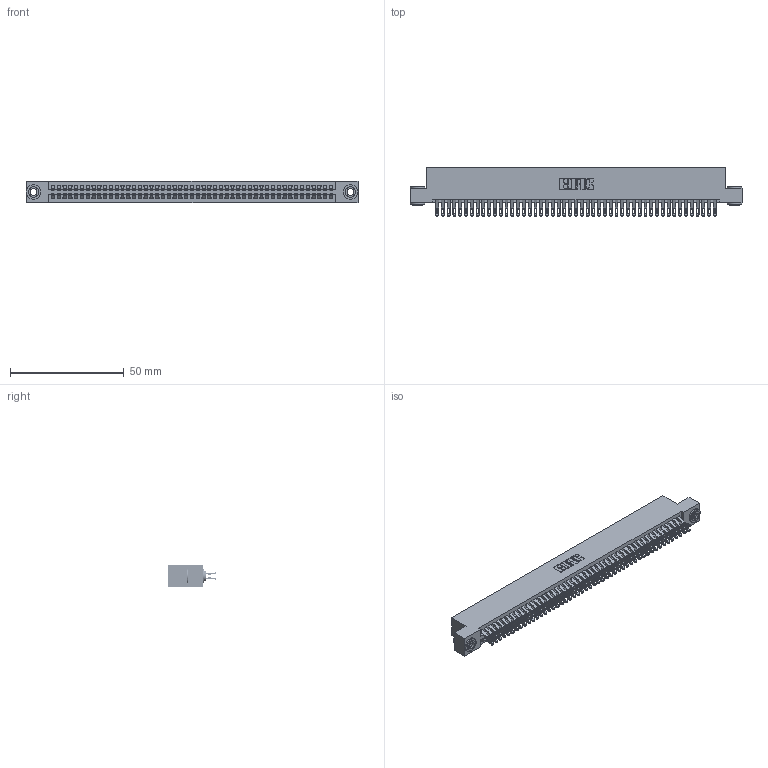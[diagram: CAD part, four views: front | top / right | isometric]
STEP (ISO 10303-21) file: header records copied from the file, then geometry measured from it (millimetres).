
FILE_DESCRIPTION (( 'STEP AP203' ), '1' );
FILE_NAME ('345-098-555-203.STEP', '2018-10-05T10:45:41', ( '' ), ( '' ), 'SwSTEP 2.0', 'SolidWorks 2016', '' );
FILE_SCHEMA (( 'CONFIG_CONTROL_DESIGN' ));
Length unit declared in the file: inch
Products named in the file (4): 345 Part_Flush Mounting Lugs - 0.156 Dia-TH; 345-098-555-203; 345-250-002_345-250-002-102; 345-292-001_555 Tail
Assembly tree (101 placements, depth 2):
  345-098-555-203
    345 Part_Flush Mounting Lugs - 0.156 Dia-TH
    345-292-001_555 Tail  x98
    345-250-002_345-250-002-102  x2
Bounding box: 145.67 x 21.13 x 9.4 mm (x, y, z)
Volume: 14519.1 mm3; surface area: 22790.7 mm2
Topology: 101 solids, 101 shells, 5652 faces, 17763 edges, 11838 vertices
Faces by surface type: plane 3128, cylinder 2516, cone 8
Entity records: 38480 total; most frequent: CARTESIAN_POINT 6453, ORIENTED_EDGE 6350, DIRECTION 5681, EDGE_CURVE 3175, LINE 2803, VECTOR 2803, VERTEX_POINT 2114, AXIS2_PLACEMENT_3D 1439
